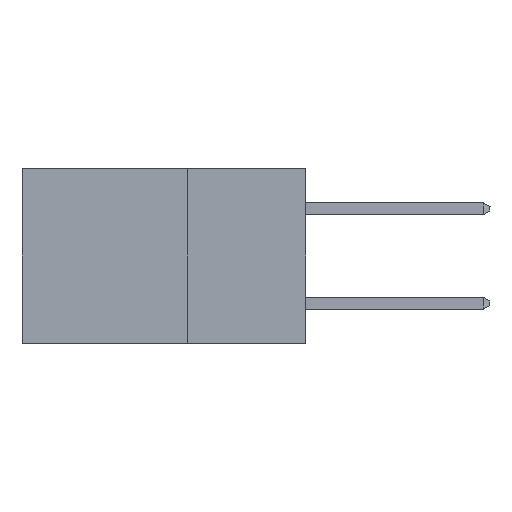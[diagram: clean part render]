
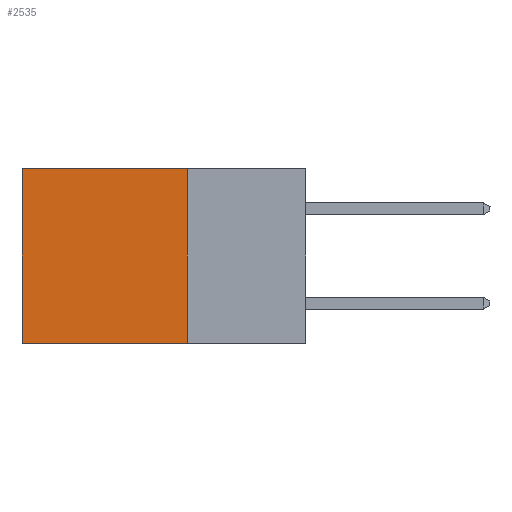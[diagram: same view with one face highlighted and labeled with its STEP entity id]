
A CAD part, left-side view. The second image highlights one B-rep face of the part: STEP entity #2535.
In plain terms, the highlighted planar face has unit normal (-1, 0, 0).
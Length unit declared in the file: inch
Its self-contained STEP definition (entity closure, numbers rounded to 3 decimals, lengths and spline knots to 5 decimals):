
#341 = CARTESIAN_POINT ( 'NONE',  ( 0.298, 0.25, 0. ) ) ;
#1125 = VERTEX_POINT ( 'NONE', #22291 ) ;
#1875 = DIRECTION ( 'NONE',  ( 1., 0., 0. ) ) ;
#1887 = VERTEX_POINT ( 'NONE', #12835 ) ;
#2535 = ADVANCED_FACE ( 'NONE', ( #11449 ), #12352, .F. ) ;
#3882 = VECTOR ( 'NONE', #5431, 39.37008 ) ;
#4070 = VERTEX_POINT ( 'NONE', #17593 ) ;
#4186 = EDGE_CURVE ( 'NONE', #19834, #4070, #4502, .T. ) ;
#4502 = LINE ( 'NONE', #16423, #22131 ) ;
#4696 = ORIENTED_EDGE ( 'NONE', *, *, #14928, .F. ) ;
#4912 = VECTOR ( 'NONE', #7340, 39.37008 ) ;
#5431 = DIRECTION ( 'NONE',  ( 0., 0., -1. ) ) ;
#6801 = ORIENTED_EDGE ( 'NONE', *, *, #16003, .F. ) ;
#7239 = DIRECTION ( 'NONE',  ( 0., 1., 0. ) ) ;
#7329 = DIRECTION ( 'NONE',  ( 0., 0., -1. ) ) ;
#7340 = DIRECTION ( 'NONE',  ( 0., 1., 0. ) ) ;
#8350 = AXIS2_PLACEMENT_3D ( 'NONE', #21185, #1875, #7329 ) ;
#8749 = LINE ( 'NONE', #341, #4912 ) ;
#9494 = CARTESIAN_POINT ( 'NONE',  ( 0.298, 0.25, -0.37 ) ) ;
#10449 = CARTESIAN_POINT ( 'NONE',  ( 0.298, 0.6, 0. ) ) ;
#11449 = FACE_OUTER_BOUND ( 'NONE', #13579, .T. ) ;
#12352 = PLANE ( 'NONE',  #8350 ) ;
#12835 = CARTESIAN_POINT ( 'NONE',  ( 0.298, 0.25, 0. ) ) ;
#12959 = VECTOR ( 'NONE', #7239, 39.37008 ) ;
#13579 = EDGE_LOOP ( 'NONE', ( #21292, #6801, #4696, #18520 ) ) ;
#14282 = CARTESIAN_POINT ( 'NONE',  ( 0.298, 0.25, 0. ) ) ;
#14622 = DIRECTION ( 'NONE',  ( 0., 0., -1. ) ) ;
#14928 = EDGE_CURVE ( 'NONE', #1887, #1125, #22313, .T. ) ;
#16003 = EDGE_CURVE ( 'NONE', #1125, #4070, #17611, .T. ) ;
#16423 = CARTESIAN_POINT ( 'NONE',  ( 0.298, 0.6, 0. ) ) ;
#16858 = EDGE_CURVE ( 'NONE', #1887, #19834, #8749, .T. ) ;
#17593 = CARTESIAN_POINT ( 'NONE',  ( 0.298, 0.6, -0.37 ) ) ;
#17611 = LINE ( 'NONE', #9494, #12959 ) ;
#18520 = ORIENTED_EDGE ( 'NONE', *, *, #16858, .T. ) ;
#19834 = VERTEX_POINT ( 'NONE', #10449 ) ;
#21185 = CARTESIAN_POINT ( 'NONE',  ( 0.298, 0.25, 0. ) ) ;
#21292 = ORIENTED_EDGE ( 'NONE', *, *, #4186, .T. ) ;
#22131 = VECTOR ( 'NONE', #14622, 39.37008 ) ;
#22291 = CARTESIAN_POINT ( 'NONE',  ( 0.298, 0.25, -0.37 ) ) ;
#22313 = LINE ( 'NONE', #14282, #3882 ) ;
